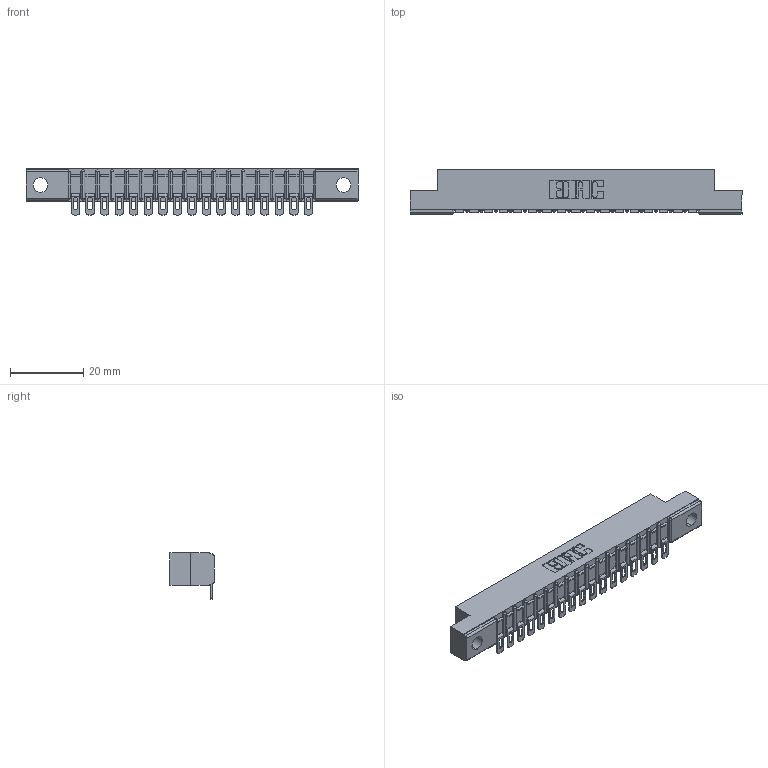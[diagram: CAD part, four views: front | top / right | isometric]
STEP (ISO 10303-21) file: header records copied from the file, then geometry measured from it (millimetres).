
FILE_DESCRIPTION (( 'STEP AP203' ), '1' );
FILE_NAME ('357-017-454-104.STEP', '2020-09-30T23:02:24', ( '' ), ( '' ), 'SwSTEP 2.0', 'SolidWorks 2020', '' );
FILE_SCHEMA (( 'CONFIG_CONTROL_DESIGN' ));
Length unit declared in the file: inch
Products named in the file (3): 357-017-454-104; 307 Part_.156 Dia Mounting Holes; 307-290-002_554
Assembly tree (18 placements, depth 2):
  357-017-454-104
    307 Part_.156 Dia Mounting Holes
    307-290-002_554  x17
Bounding box: 90.37 x 12.01 x 12.52 mm (x, y, z)
Volume: 5863.8 mm3; surface area: 10348 mm2
Topology: 18 solids, 18 shells, 1527 faces, 4660 edges, 3056 vertices
Faces by surface type: plane 866, cylinder 625, sphere 36
Entity records: 19039 total; most frequent: CARTESIAN_POINT 3212, ORIENTED_EDGE 3200, DIRECTION 3130, EDGE_CURVE 1600, VECTOR 1214, LINE 1214, VERTEX_POINT 1040, AXIS2_PLACEMENT_3D 958
